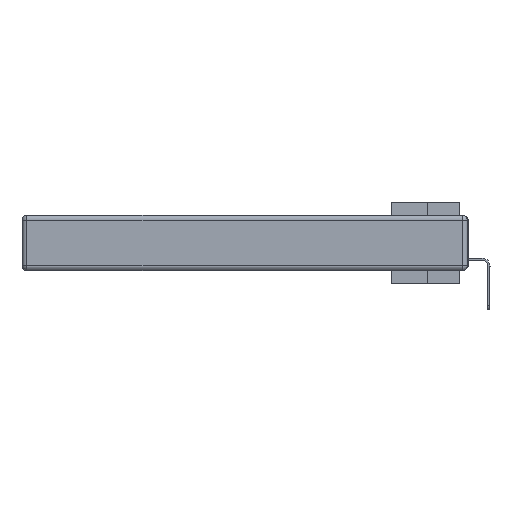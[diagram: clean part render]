
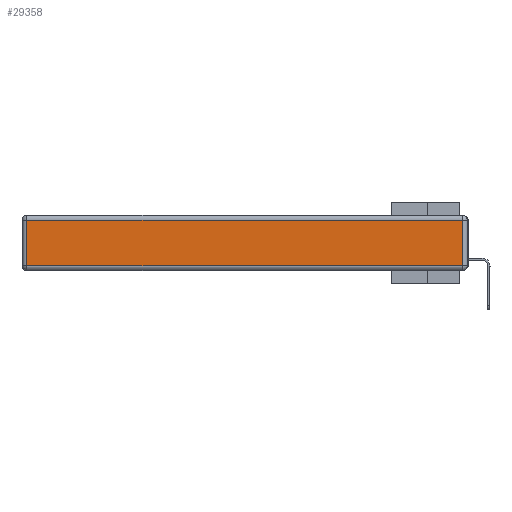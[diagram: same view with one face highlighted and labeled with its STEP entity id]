
A CAD part, left-side view. The second image highlights one B-rep face of the part: STEP entity #29358.
In plain terms, the highlighted planar face has unit normal (-1, 0, 0).
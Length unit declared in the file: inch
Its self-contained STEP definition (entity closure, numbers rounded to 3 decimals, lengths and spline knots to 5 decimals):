
#366 = CARTESIAN_POINT ( 'NONE',  ( 0., 2.72, -0.343 ) ) ;
#1446 = VECTOR ( 'NONE', #9726, 39.37008 ) ;
#2818 = CARTESIAN_POINT ( 'NONE',  ( 0., 0.03, -0.343 ) ) ;
#3001 = VERTEX_POINT ( 'NONE', #11339 ) ;
#4068 = LINE ( 'NONE', #5768, #7747 ) ;
#4359 = FACE_OUTER_BOUND ( 'NONE', #21588, .T. ) ;
#5768 = CARTESIAN_POINT ( 'NONE',  ( 0., 2.75, -0.03 ) ) ;
#7185 = EDGE_CURVE ( 'NONE', #8969, #16732, #29889, .T. ) ;
#7435 = ORIENTED_EDGE ( 'NONE', *, *, #7185, .T. ) ;
#7747 = VECTOR ( 'NONE', #28816, 39.37008 ) ;
#7908 = LINE ( 'NONE', #29429, #9737 ) ;
#8651 = CARTESIAN_POINT ( 'NONE',  ( 0., 0.03, -0.03 ) ) ;
#8969 = VERTEX_POINT ( 'NONE', #11789 ) ;
#9726 = DIRECTION ( 'NONE',  ( 0., 0., -1. ) ) ;
#9737 = VECTOR ( 'NONE', #18008, 39.37008 ) ;
#9927 = PLANE ( 'NONE',  #30006 ) ;
#10010 = ORIENTED_EDGE ( 'NONE', *, *, #11315, .T. ) ;
#10131 = DIRECTION ( 'NONE',  ( 0., 0., 1. ) ) ;
#10581 = LINE ( 'NONE', #366, #1446 ) ;
#11315 = EDGE_CURVE ( 'NONE', #3001, #8969, #7908, .T. ) ;
#11339 = CARTESIAN_POINT ( 'NONE',  ( 0., 2.72, -0.313 ) ) ;
#11789 = CARTESIAN_POINT ( 'NONE',  ( 0., 0.03, -0.313 ) ) ;
#12361 = DIRECTION ( 'NONE',  ( -1., 0., 0. ) ) ;
#13508 = EDGE_CURVE ( 'NONE', #16816, #3001, #10581, .T. ) ;
#13965 = CARTESIAN_POINT ( 'NONE',  ( 0., 2.72, -0.03 ) ) ;
#14651 = DIRECTION ( 'NONE',  ( 0., 0., 1. ) ) ;
#16732 = VERTEX_POINT ( 'NONE', #8651 ) ;
#16816 = VERTEX_POINT ( 'NONE', #13965 ) ;
#17197 = EDGE_CURVE ( 'NONE', #16732, #16816, #4068, .T. ) ;
#18008 = DIRECTION ( 'NONE',  ( 0., -1., 0. ) ) ;
#19248 = CARTESIAN_POINT ( 'NONE',  ( 0., 0., -0.343 ) ) ;
#19770 = ORIENTED_EDGE ( 'NONE', *, *, #17197, .T. ) ;
#21588 = EDGE_LOOP ( 'NONE', ( #10010, #7435, #19770, #26605 ) ) ;
#24838 = VECTOR ( 'NONE', #14651, 39.37008 ) ;
#26605 = ORIENTED_EDGE ( 'NONE', *, *, #13508, .T. ) ;
#28816 = DIRECTION ( 'NONE',  ( 0., 1., 0. ) ) ;
#29358 = ADVANCED_FACE ( 'NONE', ( #4359 ), #9927, .T. ) ;
#29429 = CARTESIAN_POINT ( 'NONE',  ( 0., 0., -0.313 ) ) ;
#29889 = LINE ( 'NONE', #2818, #24838 ) ;
#30006 = AXIS2_PLACEMENT_3D ( 'NONE', #19248, #12361, #10131 ) ;
